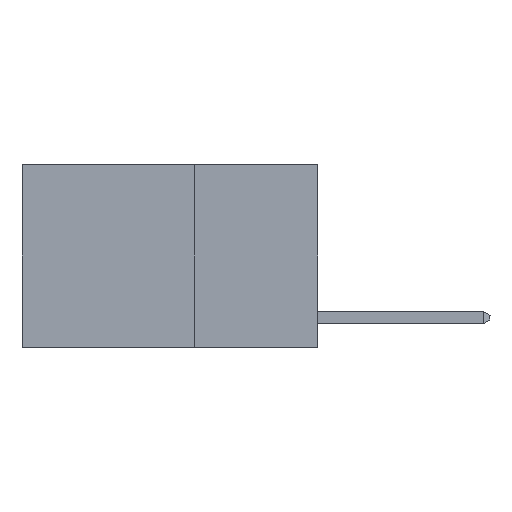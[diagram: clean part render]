
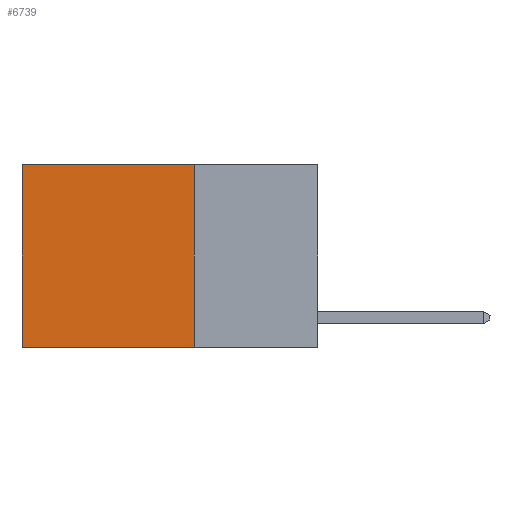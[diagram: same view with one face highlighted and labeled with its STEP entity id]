
A CAD part, left-side view. The second image highlights one B-rep face of the part: STEP entity #6739.
In plain terms, the highlighted planar face has unit normal (-1, 0, 0).
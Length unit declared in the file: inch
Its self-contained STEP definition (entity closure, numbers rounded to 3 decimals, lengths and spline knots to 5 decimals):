
#1373 = EDGE_CURVE ( 'NONE', #14620, #15194, #2345, .T. ) ;
#1429 = ORIENTED_EDGE ( 'NONE', *, *, #1373, .T. ) ;
#2345 = LINE ( 'NONE', #14186, #7357 ) ;
#2501 = DIRECTION ( 'NONE',  ( 1., 0., 0. ) ) ;
#3961 = CARTESIAN_POINT ( 'NONE',  ( 0.2625, 0.25, 0. ) ) ;
#5550 = DIRECTION ( 'NONE',  ( 0., 1., 0. ) ) ;
#6193 = EDGE_CURVE ( 'NONE', #14620, #11971, #10517, .T. ) ;
#6716 = VERTEX_POINT ( 'NONE', #20581 ) ;
#6739 = ADVANCED_FACE ( 'NONE', ( #14127 ), #9398, .F. ) ;
#6978 = VECTOR ( 'NONE', #16748, 39.37008 ) ;
#7318 = LINE ( 'NONE', #14010, #18571 ) ;
#7357 = VECTOR ( 'NONE', #5550, 39.37008 ) ;
#8499 = CARTESIAN_POINT ( 'NONE',  ( 0.2625, 0.25, 0. ) ) ;
#9086 = DIRECTION ( 'NONE',  ( 0., 0., -1. ) ) ;
#9319 = EDGE_CURVE ( 'NONE', #11971, #6716, #14984, .T. ) ;
#9398 = PLANE ( 'NONE',  #14105 ) ;
#9487 = EDGE_LOOP ( 'NONE', ( #15389, #14726, #17838, #1429 ) ) ;
#10517 = LINE ( 'NONE', #3961, #14499 ) ;
#10848 = EDGE_CURVE ( 'NONE', #15194, #6716, #7318, .T. ) ;
#10922 = DIRECTION ( 'NONE',  ( 0., 0., -1. ) ) ;
#11971 = VERTEX_POINT ( 'NONE', #16899 ) ;
#13930 = DIRECTION ( 'NONE',  ( 0., 0., -1. ) ) ;
#14010 = CARTESIAN_POINT ( 'NONE',  ( 0.2625, 0.6, 0. ) ) ;
#14105 = AXIS2_PLACEMENT_3D ( 'NONE', #17517, #2501, #9086 ) ;
#14127 = FACE_OUTER_BOUND ( 'NONE', #9487, .T. ) ;
#14186 = CARTESIAN_POINT ( 'NONE',  ( 0.2625, 0.25, 0. ) ) ;
#14499 = VECTOR ( 'NONE', #13930, 39.37008 ) ;
#14620 = VERTEX_POINT ( 'NONE', #8499 ) ;
#14726 = ORIENTED_EDGE ( 'NONE', *, *, #9319, .F. ) ;
#14984 = LINE ( 'NONE', #16861, #6978 ) ;
#15194 = VERTEX_POINT ( 'NONE', #18545 ) ;
#15389 = ORIENTED_EDGE ( 'NONE', *, *, #10848, .T. ) ;
#16748 = DIRECTION ( 'NONE',  ( 0., 1., 0. ) ) ;
#16861 = CARTESIAN_POINT ( 'NONE',  ( 0.2625, 0.25, -0.37 ) ) ;
#16899 = CARTESIAN_POINT ( 'NONE',  ( 0.2625, 0.25, -0.37 ) ) ;
#17517 = CARTESIAN_POINT ( 'NONE',  ( 0.2625, 0.25, 0. ) ) ;
#17838 = ORIENTED_EDGE ( 'NONE', *, *, #6193, .F. ) ;
#18545 = CARTESIAN_POINT ( 'NONE',  ( 0.2625, 0.6, 0. ) ) ;
#18571 = VECTOR ( 'NONE', #10922, 39.37008 ) ;
#20581 = CARTESIAN_POINT ( 'NONE',  ( 0.2625, 0.6, -0.37 ) ) ;
